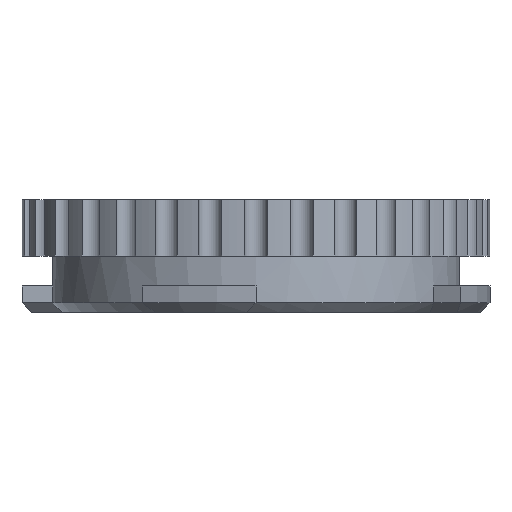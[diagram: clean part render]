
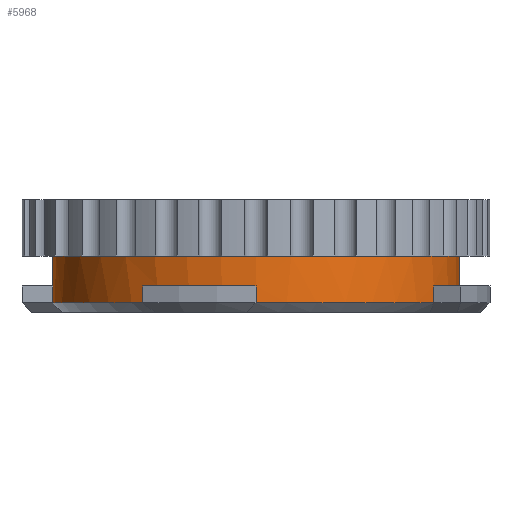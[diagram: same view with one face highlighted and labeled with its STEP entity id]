
A CAD part, front view. The second image highlights one B-rep face of the part: STEP entity #5968.
In plain terms, the highlighted cylindrical face has radius 13.787 mm (diameter 27.575 mm), a partial arc.
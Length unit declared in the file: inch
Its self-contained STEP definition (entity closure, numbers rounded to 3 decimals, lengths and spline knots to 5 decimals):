
#59 = CARTESIAN_POINT ( 'NONE',  ( 0., -0.54281, 0.02461 ) ) ;
#90 = CARTESIAN_POINT ( 'NONE',  ( 0.54281, 0., 0.15 ) ) ;
#286 = DIRECTION ( 'NONE',  ( 0., 0., -1. ) ) ;
#324 = LINE ( 'NONE', #5475, #10829 ) ;
#477 = EDGE_LOOP ( 'NONE', ( #1242, #7121, #10299, #10561, #6465, #10432, #9628, #3946, #8391, #12171, #7428 ) ) ;
#606 = DIRECTION ( 'NONE',  ( 0., 0., 1. ) ) ;
#897 = CYLINDRICAL_SURFACE ( 'NONE', #4599, 0.54281 ) ;
#1058 = EDGE_CURVE ( 'NONE', #3967, #6150, #12763, .T. ) ;
#1242 = ORIENTED_EDGE ( 'NONE', *, *, #8300, .F. ) ;
#1304 = AXIS2_PLACEMENT_3D ( 'NONE', #11606, #9619, #3630 ) ;
#1316 = EDGE_CURVE ( 'NONE', #13109, #9296, #2912, .T. ) ;
#1426 = DIRECTION ( 'NONE',  ( 1., 0., 0. ) ) ;
#1484 = VERTEX_POINT ( 'NONE', #7517 ) ;
#1533 = CARTESIAN_POINT ( 'NONE',  ( 0.47476, -0.26316, 0.15 ) ) ;
#1618 = DIRECTION ( 'NONE',  ( -1., 0., 0. ) ) ;
#1653 = CARTESIAN_POINT ( 'NONE',  ( -0.54281, 0., 0.15 ) ) ;
#1784 = LINE ( 'NONE', #90, #8781 ) ;
#1897 = VECTOR ( 'NONE', #11962, 39.37008 ) ;
#1900 = CARTESIAN_POINT ( 'NONE',  ( -0.26316, -0.47476, 0.15 ) ) ;
#2137 = EDGE_CURVE ( 'NONE', #1484, #3638, #8428, .T. ) ;
#2218 = EDGE_CURVE ( 'NONE', #10267, #4115, #11274, .T. ) ;
#2334 = DIRECTION ( 'NONE',  ( 0., 0., 1. ) ) ;
#2368 = CARTESIAN_POINT ( 'NONE',  ( 0.47476, -0.26316, 0.07 ) ) ;
#2421 = LINE ( 'NONE', #1533, #10222 ) ;
#2490 = CARTESIAN_POINT ( 'NONE',  ( 0.47476, -0.26316, 0.02461 ) ) ;
#2546 = CARTESIAN_POINT ( 'NONE',  ( 0., -0.54281, 0.07 ) ) ;
#2618 = EDGE_CURVE ( 'NONE', #9296, #1484, #5559, .T. ) ;
#2898 = DIRECTION ( 'NONE',  ( 1., 0., 0. ) ) ;
#2912 = LINE ( 'NONE', #6497, #7846 ) ;
#3521 = DIRECTION ( 'NONE',  ( 0., 0., 1. ) ) ;
#3557 = CARTESIAN_POINT ( 'NONE',  ( 0., 0., 0.02461 ) ) ;
#3630 = DIRECTION ( 'NONE',  ( 0., -1., 0. ) ) ;
#3638 = VERTEX_POINT ( 'NONE', #12900 ) ;
#3651 = CIRCLE ( 'NONE', #9504, 0.54281 ) ;
#3946 = ORIENTED_EDGE ( 'NONE', *, *, #8780, .T. ) ;
#3967 = VERTEX_POINT ( 'NONE', #11358 ) ;
#4115 = VERTEX_POINT ( 'NONE', #2490 ) ;
#4599 = AXIS2_PLACEMENT_3D ( 'NONE', #5716, #10659, #1618 ) ;
#4604 = DIRECTION ( 'NONE',  ( 0., 0., 1. ) ) ;
#4939 = CARTESIAN_POINT ( 'NONE',  ( 0., 0., 0.02461 ) ) ;
#5475 = CARTESIAN_POINT ( 'NONE',  ( 0., -0.54281, 0.15 ) ) ;
#5559 = LINE ( 'NONE', #1653, #1897 ) ;
#5629 = CARTESIAN_POINT ( 'NONE',  ( 0.54281, 0., 0.07 ) ) ;
#5716 = CARTESIAN_POINT ( 'NONE',  ( 0., 0., 0.15 ) ) ;
#5968 = ADVANCED_FACE ( 'NONE', ( #12028 ), #897, .T. ) ;
#6018 = AXIS2_PLACEMENT_3D ( 'NONE', #3557, #4604, #1426 ) ;
#6039 = DIRECTION ( 'NONE',  ( 0., 0., 1. ) ) ;
#6150 = VERTEX_POINT ( 'NONE', #2546 ) ;
#6198 = LINE ( 'NONE', #1900, #8576 ) ;
#6465 = ORIENTED_EDGE ( 'NONE', *, *, #2137, .T. ) ;
#6497 = CARTESIAN_POINT ( 'NONE',  ( -0.54281, 0., 0.15 ) ) ;
#6589 = AXIS2_PLACEMENT_3D ( 'NONE', #8976, #13099, #2898 ) ;
#7121 = ORIENTED_EDGE ( 'NONE', *, *, #11691, .F. ) ;
#7428 = ORIENTED_EDGE ( 'NONE', *, *, #12580, .T. ) ;
#7517 = CARTESIAN_POINT ( 'NONE',  ( -0.54281, 0., 0.02461 ) ) ;
#7846 = VECTOR ( 'NONE', #11553, 39.37008 ) ;
#8280 = CIRCLE ( 'NONE', #6589, 0.54281 ) ;
#8300 = EDGE_CURVE ( 'NONE', #10569, #8489, #1784, .T. ) ;
#8391 = ORIENTED_EDGE ( 'NONE', *, *, #2218, .T. ) ;
#8428 = CIRCLE ( 'NONE', #9154, 0.54281 ) ;
#8489 = VERTEX_POINT ( 'NONE', #5629 ) ;
#8576 = VECTOR ( 'NONE', #6039, 39.37008 ) ;
#8780 = EDGE_CURVE ( 'NONE', #6150, #10267, #324, .T. ) ;
#8781 = VECTOR ( 'NONE', #10228, 39.37008 ) ;
#8976 = CARTESIAN_POINT ( 'NONE',  ( 0., 0., 0.15 ) ) ;
#8979 = CARTESIAN_POINT ( 'NONE',  ( -0.54281, 0., 0.15 ) ) ;
#9154 = AXIS2_PLACEMENT_3D ( 'NONE', #4939, #2334, #10455 ) ;
#9296 = VERTEX_POINT ( 'NONE', #10336 ) ;
#9504 = AXIS2_PLACEMENT_3D ( 'NONE', #9664, #606, #11641 ) ;
#9619 = DIRECTION ( 'NONE',  ( 0., 0., 1. ) ) ;
#9628 = ORIENTED_EDGE ( 'NONE', *, *, #1058, .T. ) ;
#9664 = CARTESIAN_POINT ( 'NONE',  ( 0., 0., 0.07 ) ) ;
#10222 = VECTOR ( 'NONE', #3521, 39.37008 ) ;
#10228 = DIRECTION ( 'NONE',  ( 0., 0., -1. ) ) ;
#10267 = VERTEX_POINT ( 'NONE', #59 ) ;
#10299 = ORIENTED_EDGE ( 'NONE', *, *, #1316, .T. ) ;
#10336 = CARTESIAN_POINT ( 'NONE',  ( -0.54281, 0., 0.07 ) ) ;
#10432 = ORIENTED_EDGE ( 'NONE', *, *, #12267, .T. ) ;
#10455 = DIRECTION ( 'NONE',  ( 1., 0., 0. ) ) ;
#10506 = EDGE_CURVE ( 'NONE', #4115, #12486, #2421, .T. ) ;
#10561 = ORIENTED_EDGE ( 'NONE', *, *, #2618, .T. ) ;
#10569 = VERTEX_POINT ( 'NONE', #12621 ) ;
#10659 = DIRECTION ( 'NONE',  ( 0., 0., -1. ) ) ;
#10829 = VECTOR ( 'NONE', #286, 39.37008 ) ;
#11274 = CIRCLE ( 'NONE', #6018, 0.54281 ) ;
#11358 = CARTESIAN_POINT ( 'NONE',  ( -0.26316, -0.47476, 0.07 ) ) ;
#11553 = DIRECTION ( 'NONE',  ( 0., 0., -1. ) ) ;
#11606 = CARTESIAN_POINT ( 'NONE',  ( 0., 0., 0.07 ) ) ;
#11641 = DIRECTION ( 'NONE',  ( 1., 0., 0. ) ) ;
#11691 = EDGE_CURVE ( 'NONE', #13109, #10569, #8280, .T. ) ;
#11962 = DIRECTION ( 'NONE',  ( 0., 0., -1. ) ) ;
#12028 = FACE_OUTER_BOUND ( 'NONE', #477, .T. ) ;
#12171 = ORIENTED_EDGE ( 'NONE', *, *, #10506, .T. ) ;
#12267 = EDGE_CURVE ( 'NONE', #3638, #3967, #6198, .T. ) ;
#12486 = VERTEX_POINT ( 'NONE', #2368 ) ;
#12580 = EDGE_CURVE ( 'NONE', #12486, #8489, #3651, .T. ) ;
#12621 = CARTESIAN_POINT ( 'NONE',  ( 0.54281, 0., 0.15 ) ) ;
#12763 = CIRCLE ( 'NONE', #1304, 0.54281 ) ;
#12900 = CARTESIAN_POINT ( 'NONE',  ( -0.26316, -0.47476, 0.02461 ) ) ;
#13099 = DIRECTION ( 'NONE',  ( 0., 0., 1. ) ) ;
#13109 = VERTEX_POINT ( 'NONE', #8979 ) ;
